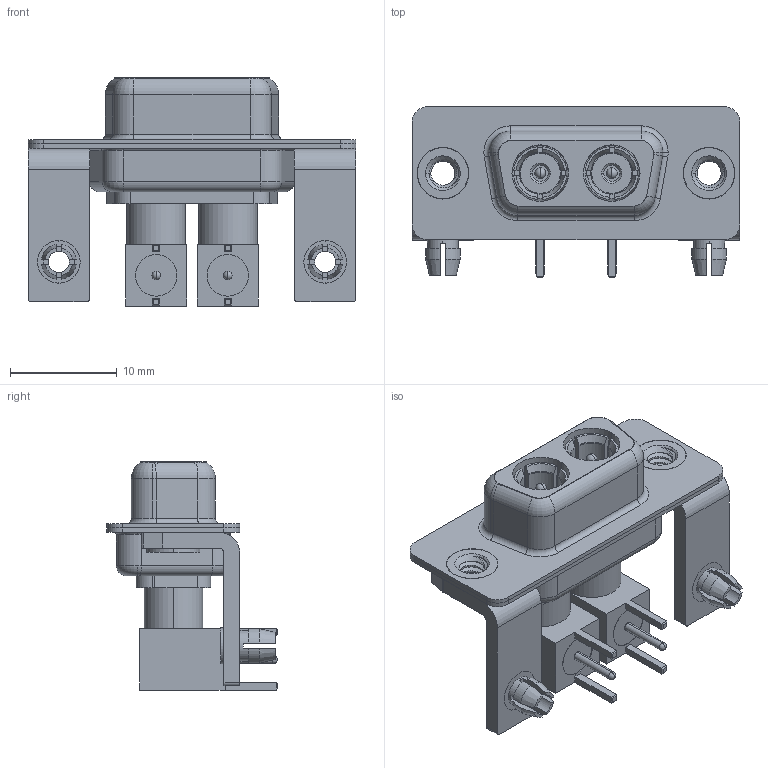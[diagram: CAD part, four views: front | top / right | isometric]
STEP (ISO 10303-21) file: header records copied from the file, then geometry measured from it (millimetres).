
FILE_DESCRIPTION (( 'STEP AP203' ), '1' );
FILE_NAME ('630-2W2-640-7T3.STEP', '2022-05-26T19:57:41', ( '' ), ( '' ), 'SwSTEP 2.0', 'SolidWorks 2020', '' );
FILE_SCHEMA (( 'CONFIG_CONTROL_DESIGN' ));
Length unit declared in the file: millimetre
Products named in the file (15): Locking Collar; 630Combo Shell Front_09 Contacts; 630Combo Stabilizer Bracket; Co-Ax Plug Assy_RA; 630Combo Housing_2W2; 630Combo Threaded Rivet_3; Co-Ax Plug_RA PC Tail; Insulator Pin_Straight PC Tail; 630Combo Shell Rear_09 Contacts; Pin_RA; RA Back Shell; Insulator RA Pin; 630Combo Board Lock; 630-2W2-640-7T3
Assembly tree (23 placements, depth 3):
  630-2W2-640-7T3
    630Combo Housing_2W2
    630Combo Shell Front_09 Contacts
    630Combo Shell Rear_09 Contacts
    630Combo Threaded Rivet_3  x2
    630Combo Stabilizer Bracket  x2
    630Combo Board Lock  x2
    Co-Ax Plug Assy_RA
      Co-Ax Plug_RA PC Tail
      Insulator Pin_Straight PC Tail
      Pin_RA
      Locking Collar
      RA Back Shell
      Insulator RA Pin
    Co-Ax Plug Assy_RA
      Co-Ax Plug_RA PC Tail
      Insulator Pin_Straight PC Tail
      Pin_RA
      Locking Collar
      RA Back Shell
      Insulator RA Pin
Bounding box: 30.8 x 16 x 21.41 mm (x, y, z)
Volume: 2441.8 mm3; surface area: 6433.5 mm2
Topology: 21 solids, 21 shells, 747 faces, 1837 edges, 1159 vertices
Faces by surface type: cylinder 317, plane 269, cone 76, torus 69, bspline 8, sphere 8
Entity records: 17894 total; most frequent: CARTESIAN_POINT 4319, DIRECTION 2634, ORIENTED_EDGE 2360, EDGE_CURVE 1180, AXIS2_PLACEMENT_3D 1050, VERTEX_POINT 747, EDGE_LOOP 545, CIRCLE 541
